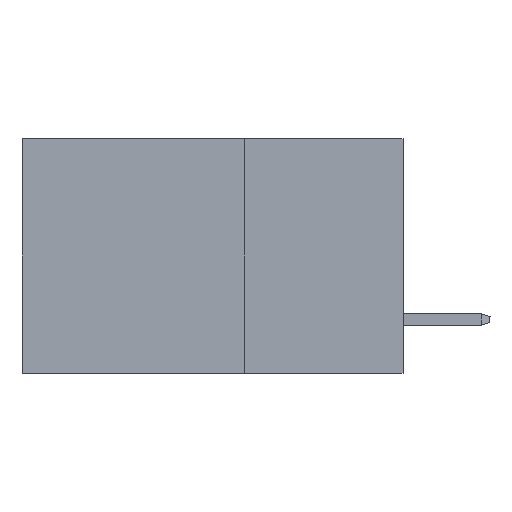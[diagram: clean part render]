
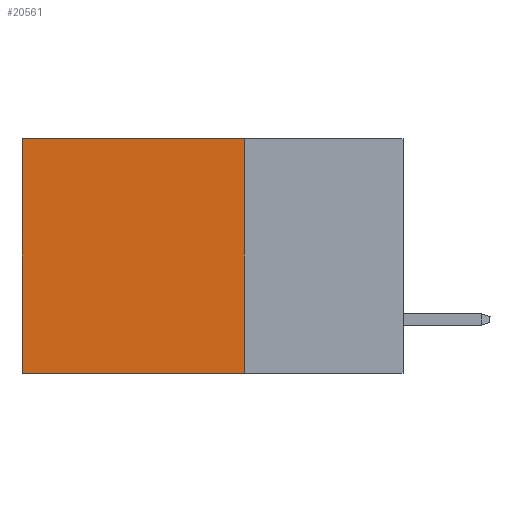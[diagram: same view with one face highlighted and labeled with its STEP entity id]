
A CAD part, left-side view. The second image highlights one B-rep face of the part: STEP entity #20561.
In plain terms, the highlighted planar face has unit normal (-1, 0, 0).
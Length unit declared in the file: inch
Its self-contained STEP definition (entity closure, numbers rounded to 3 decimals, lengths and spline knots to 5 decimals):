
#5572 = CARTESIAN_POINT ( 'NONE',  ( 0.2875, 0.6, -0.37 ) ) ;
#7072 = VECTOR ( 'NONE', #39915, 39.37008 ) ;
#7710 = AXIS2_PLACEMENT_3D ( 'NONE', #33658, #46401, #38581 ) ;
#8376 = DIRECTION ( 'NONE',  ( 0., 0., -1. ) ) ;
#8726 = CARTESIAN_POINT ( 'NONE',  ( 0.2875, 0.25, -0.37 ) ) ;
#12591 = ORIENTED_EDGE ( 'NONE', *, *, #40760, .F. ) ;
#13112 = EDGE_LOOP ( 'NONE', ( #27684, #37399, #12591, #18457 ) ) ;
#14678 = FACE_OUTER_BOUND ( 'NONE', #13112, .T. ) ;
#17262 = CARTESIAN_POINT ( 'NONE',  ( 0.2875, 0.25, 0. ) ) ;
#17712 = VERTEX_POINT ( 'NONE', #30204 ) ;
#18457 = ORIENTED_EDGE ( 'NONE', *, *, #41801, .T. ) ;
#19482 = EDGE_CURVE ( 'NONE', #17712, #36424, #25288, .T. ) ;
#20154 = VECTOR ( 'NONE', #8376, 39.37008 ) ;
#20561 = ADVANCED_FACE ( 'NONE', ( #14678 ), #38853, .F. ) ;
#20896 = CARTESIAN_POINT ( 'NONE',  ( 0.2875, 0.6, 0. ) ) ;
#23815 = VECTOR ( 'NONE', #32164, 39.37008 ) ;
#25018 = CARTESIAN_POINT ( 'NONE',  ( 0.2875, 0.25, -0.37 ) ) ;
#25288 = LINE ( 'NONE', #20896, #20154 ) ;
#26259 = CARTESIAN_POINT ( 'NONE',  ( 0.2875, 0.25, 0. ) ) ;
#27684 = ORIENTED_EDGE ( 'NONE', *, *, #19482, .T. ) ;
#30204 = CARTESIAN_POINT ( 'NONE',  ( 0.2875, 0.6, 0. ) ) ;
#31903 = LINE ( 'NONE', #8726, #23815 ) ;
#32164 = DIRECTION ( 'NONE',  ( 0., 1., 0. ) ) ;
#33658 = CARTESIAN_POINT ( 'NONE',  ( 0.2875, 0.25, 0. ) ) ;
#34393 = VECTOR ( 'NONE', #42132, 39.37008 ) ;
#36424 = VERTEX_POINT ( 'NONE', #5572 ) ;
#36511 = VERTEX_POINT ( 'NONE', #45624 ) ;
#37007 = LINE ( 'NONE', #17262, #7072 ) ;
#37399 = ORIENTED_EDGE ( 'NONE', *, *, #43339, .F. ) ;
#38581 = DIRECTION ( 'NONE',  ( 0., 0., -1. ) ) ;
#38853 = PLANE ( 'NONE',  #7710 ) ;
#39915 = DIRECTION ( 'NONE',  ( 0., 1., 0. ) ) ;
#40760 = EDGE_CURVE ( 'NONE', #36511, #50601, #46299, .T. ) ;
#41801 = EDGE_CURVE ( 'NONE', #36511, #17712, #37007, .T. ) ;
#42132 = DIRECTION ( 'NONE',  ( 0., 0., -1. ) ) ;
#43339 = EDGE_CURVE ( 'NONE', #50601, #36424, #31903, .T. ) ;
#45624 = CARTESIAN_POINT ( 'NONE',  ( 0.2875, 0.25, 0. ) ) ;
#46299 = LINE ( 'NONE', #26259, #34393 ) ;
#46401 = DIRECTION ( 'NONE',  ( 1., 0., 0. ) ) ;
#50601 = VERTEX_POINT ( 'NONE', #25018 ) ;
